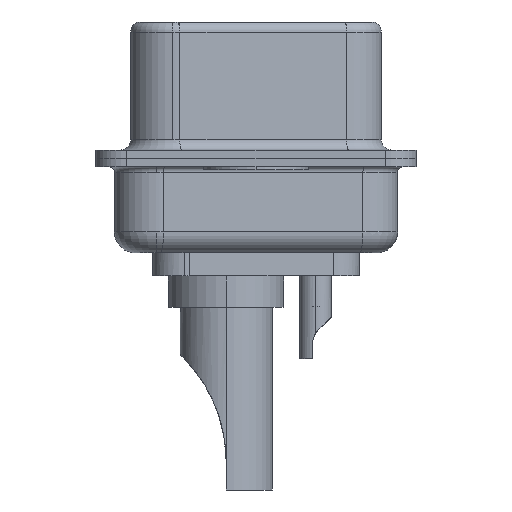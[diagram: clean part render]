
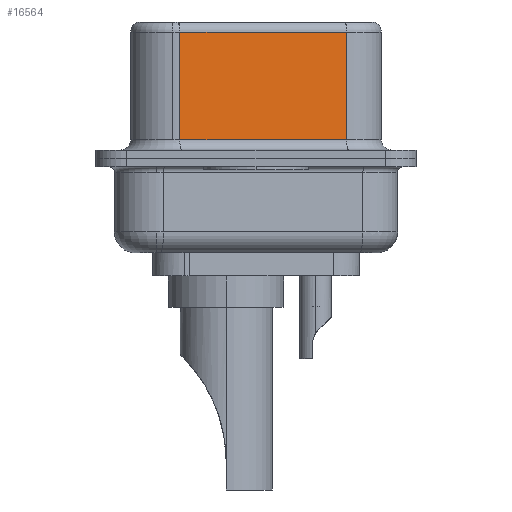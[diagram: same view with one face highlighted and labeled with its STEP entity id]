
A CAD part, left-side view. The second image highlights one B-rep face of the part: STEP entity #16564.
In plain terms, the highlighted planar face has unit normal (-0.985, -0.174, 0).
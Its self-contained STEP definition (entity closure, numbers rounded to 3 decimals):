
#634 = EDGE_CURVE ( 'NONE', #22205, #21734, #24005, .T. ) ;
#2985 = CARTESIAN_POINT ( 'NONE',  ( 5.132, -4.322, 0.9 ) ) ;
#3626 = VECTOR ( 'NONE', #19638, 1000. ) ;
#3837 = CARTESIAN_POINT ( 'NONE',  ( 3.73, 3.628, 6.52 ) ) ;
#5071 = EDGE_CURVE ( 'NONE', #12037, #22205, #12566, .T. ) ;
#5495 = ORIENTED_EDGE ( 'NONE', *, *, #11416, .F. ) ;
#6797 = DIRECTION ( 'NONE',  ( 0., 0., -1. ) ) ;
#6859 = VECTOR ( 'NONE', #22519, 1000. ) ;
#7734 = FACE_OUTER_BOUND ( 'NONE', #19788, .T. ) ;
#8585 = DIRECTION ( 'NONE',  ( 0.985, 0.174, 0. ) ) ;
#9396 = VECTOR ( 'NONE', #6797, 1000. ) ;
#11189 = CARTESIAN_POINT ( 'NONE',  ( 3.73, 3.628, 6.02 ) ) ;
#11416 = EDGE_CURVE ( 'NONE', #12037, #21006, #14540, .T. ) ;
#12037 = VERTEX_POINT ( 'NONE', #16189 ) ;
#12566 = LINE ( 'NONE', #22241, #6859 ) ;
#12735 = EDGE_CURVE ( 'NONE', #21734, #21006, #13920, .T. ) ;
#13920 = LINE ( 'NONE', #2985, #23534 ) ;
#14540 = LINE ( 'NONE', #20154, #9396 ) ;
#16189 = CARTESIAN_POINT ( 'NONE',  ( 5.132, -4.322, 6.02 ) ) ;
#16251 = PLANE ( 'NONE',  #24130 ) ;
#16564 = ADVANCED_FACE ( 'NONE', ( #7734 ), #16251, .F. ) ;
#16978 = CARTESIAN_POINT ( 'NONE',  ( 5.132, -4.322, 0.9 ) ) ;
#19383 = ORIENTED_EDGE ( 'NONE', *, *, #634, .T. ) ;
#19638 = DIRECTION ( 'NONE',  ( 0., 0., -1. ) ) ;
#19788 = EDGE_LOOP ( 'NONE', ( #5495, #20879, #19383, #24815 ) ) ;
#20154 = CARTESIAN_POINT ( 'NONE',  ( 5.132, -4.322, 6.52 ) ) ;
#20266 = DIRECTION ( 'NONE',  ( 0.174, -0.985, 0. ) ) ;
#20879 = ORIENTED_EDGE ( 'NONE', *, *, #5071, .T. ) ;
#21006 = VERTEX_POINT ( 'NONE', #16978 ) ;
#21734 = VERTEX_POINT ( 'NONE', #23238 ) ;
#21987 = DIRECTION ( 'NONE',  ( -0.174, 0.985, 0. ) ) ;
#22205 = VERTEX_POINT ( 'NONE', #11189 ) ;
#22241 = CARTESIAN_POINT ( 'NONE',  ( 5.132, -4.322, 6.02 ) ) ;
#22519 = DIRECTION ( 'NONE',  ( -0.174, 0.985, 0. ) ) ;
#23238 = CARTESIAN_POINT ( 'NONE',  ( 3.73, 3.628, 0.9 ) ) ;
#23534 = VECTOR ( 'NONE', #20266, 1000. ) ;
#23875 = CARTESIAN_POINT ( 'NONE',  ( 5.132, -4.322, 6.52 ) ) ;
#24005 = LINE ( 'NONE', #3837, #3626 ) ;
#24130 = AXIS2_PLACEMENT_3D ( 'NONE', #23875, #8585, #21987 ) ;
#24815 = ORIENTED_EDGE ( 'NONE', *, *, #12735, .T. ) ;
